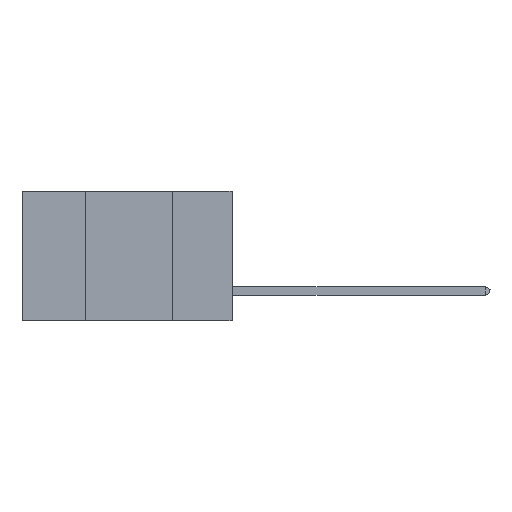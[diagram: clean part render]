
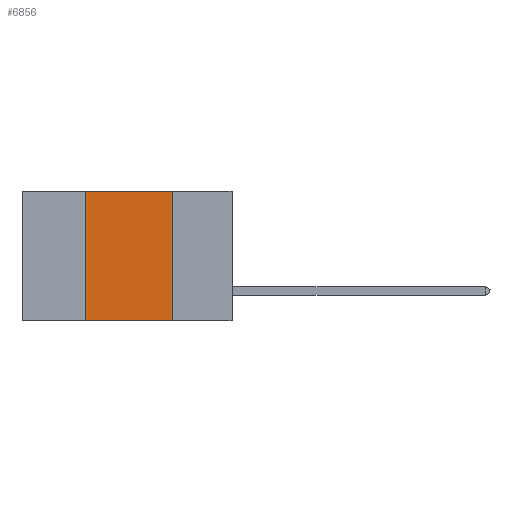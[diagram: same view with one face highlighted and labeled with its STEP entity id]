
A CAD part, left-side view. The second image highlights one B-rep face of the part: STEP entity #6856.
In plain terms, the highlighted planar face has unit normal (-1, 0, 0).
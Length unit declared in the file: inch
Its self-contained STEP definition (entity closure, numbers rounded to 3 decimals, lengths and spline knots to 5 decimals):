
#1725 = VECTOR ( 'NONE', #9839, 39.37008 ) ;
#2230 = VERTEX_POINT ( 'NONE', #13012 ) ;
#2398 = EDGE_CURVE ( 'NONE', #2230, #16642, #17620, .T. ) ;
#2680 = DIRECTION ( 'NONE',  ( 0., 0., -1. ) ) ;
#3164 = AXIS2_PLACEMENT_3D ( 'NONE', #11052, #14139, #12766 ) ;
#3461 = CARTESIAN_POINT ( 'NONE',  ( 0., 0.42, 0. ) ) ;
#4052 = CARTESIAN_POINT ( 'NONE',  ( 0., 0.17, 0. ) ) ;
#4055 = ORIENTED_EDGE ( 'NONE', *, *, #13845, .F. ) ;
#6852 = CARTESIAN_POINT ( 'NONE',  ( 0., 0.6, -0.37 ) ) ;
#6856 = ADVANCED_FACE ( 'NONE', ( #16309 ), #12696, .F. ) ;
#7330 = VERTEX_POINT ( 'NONE', #9204 ) ;
#7503 = LINE ( 'NONE', #4052, #17060 ) ;
#9177 = LINE ( 'NONE', #18301, #19227 ) ;
#9204 = CARTESIAN_POINT ( 'NONE',  ( 0., 0.17, 0. ) ) ;
#9839 = DIRECTION ( 'NONE',  ( 0., -1., 0. ) ) ;
#11046 = DIRECTION ( 'NONE',  ( 0., 0., 1. ) ) ;
#11052 = CARTESIAN_POINT ( 'NONE',  ( 0., 0.6, 0. ) ) ;
#11256 = ORIENTED_EDGE ( 'NONE', *, *, #2398, .T. ) ;
#11484 = ORIENTED_EDGE ( 'NONE', *, *, #17519, .F. ) ;
#12447 = VERTEX_POINT ( 'NONE', #3461 ) ;
#12510 = VECTOR ( 'NONE', #15452, 39.37008 ) ;
#12696 = PLANE ( 'NONE',  #3164 ) ;
#12766 = DIRECTION ( 'NONE',  ( 0., 0., -1. ) ) ;
#13012 = CARTESIAN_POINT ( 'NONE',  ( 0., 0.42, -0.37 ) ) ;
#13845 = EDGE_CURVE ( 'NONE', #7330, #16642, #7503, .T. ) ;
#14139 = DIRECTION ( 'NONE',  ( 1., 0., 0. ) ) ;
#14633 = LINE ( 'NONE', #18680, #12510 ) ;
#15268 = EDGE_LOOP ( 'NONE', ( #4055, #11484, #17505, #11256 ) ) ;
#15452 = DIRECTION ( 'NONE',  ( 0., -1., 0. ) ) ;
#16307 = CARTESIAN_POINT ( 'NONE',  ( 0., 0.17, -0.37 ) ) ;
#16309 = FACE_OUTER_BOUND ( 'NONE', #15268, .T. ) ;
#16642 = VERTEX_POINT ( 'NONE', #16307 ) ;
#17060 = VECTOR ( 'NONE', #2680, 39.37008 ) ;
#17505 = ORIENTED_EDGE ( 'NONE', *, *, #19342, .F. ) ;
#17519 = EDGE_CURVE ( 'NONE', #12447, #7330, #14633, .T. ) ;
#17620 = LINE ( 'NONE', #6852, #1725 ) ;
#18301 = CARTESIAN_POINT ( 'NONE',  ( 0., 0.42, 0. ) ) ;
#18680 = CARTESIAN_POINT ( 'NONE',  ( 0., 0.6, 0. ) ) ;
#19227 = VECTOR ( 'NONE', #11046, 39.37008 ) ;
#19342 = EDGE_CURVE ( 'NONE', #2230, #12447, #9177, .T. ) ;
